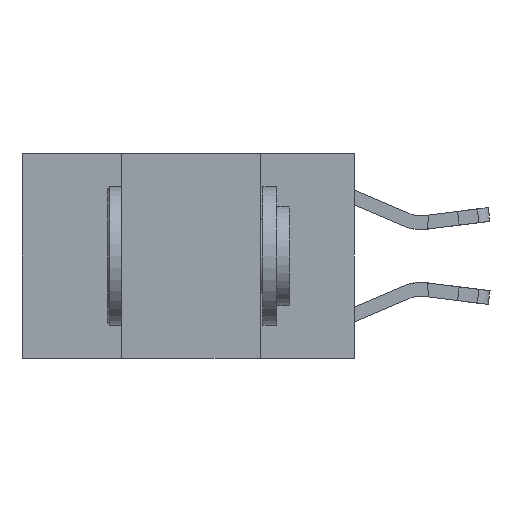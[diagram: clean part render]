
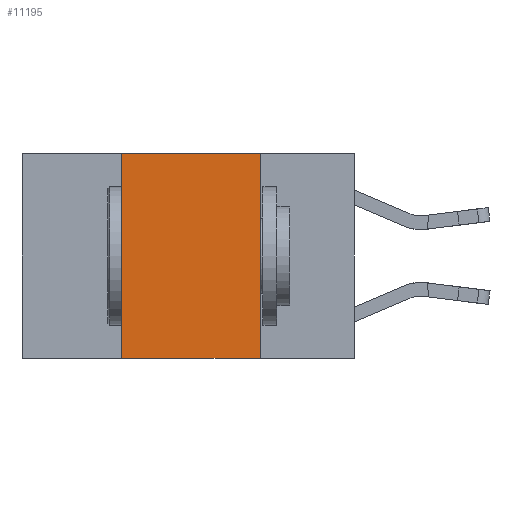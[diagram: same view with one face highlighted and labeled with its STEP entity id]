
A CAD part, left-side view. The second image highlights one B-rep face of the part: STEP entity #11195.
In plain terms, the highlighted planar face has unit normal (-1, 0, 0).
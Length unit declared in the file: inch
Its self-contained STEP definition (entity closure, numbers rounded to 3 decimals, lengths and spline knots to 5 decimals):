
#522 = CARTESIAN_POINT ( 'NONE',  ( 0., 0.42, -0.37 ) ) ;
#808 = VECTOR ( 'NONE', #12189, 39.37008 ) ;
#1566 = EDGE_CURVE ( 'NONE', #13893, #15025, #16848, .T. ) ;
#1718 = DIRECTION ( 'NONE',  ( 0., -1., 0. ) ) ;
#2200 = VECTOR ( 'NONE', #12723, 39.37008 ) ;
#2307 = ORIENTED_EDGE ( 'NONE', *, *, #5535, .F. ) ;
#2450 = EDGE_LOOP ( 'NONE', ( #11611, #2307, #12212, #3860 ) ) ;
#3753 = CARTESIAN_POINT ( 'NONE',  ( 0., 0.42, 0. ) ) ;
#3777 = DIRECTION ( 'NONE',  ( 0., 0., 1. ) ) ;
#3816 = EDGE_CURVE ( 'NONE', #8434, #16528, #4394, .T. ) ;
#3860 = ORIENTED_EDGE ( 'NONE', *, *, #13163, .T. ) ;
#4394 = LINE ( 'NONE', #14783, #808 ) ;
#5535 = EDGE_CURVE ( 'NONE', #15025, #8434, #9265, .T. ) ;
#6789 = PLANE ( 'NONE',  #6820 ) ;
#6820 = AXIS2_PLACEMENT_3D ( 'NONE', #10739, #16024, #8118 ) ;
#7435 = CARTESIAN_POINT ( 'NONE',  ( 0., 0.6, 0. ) ) ;
#8118 = DIRECTION ( 'NONE',  ( 0., 0., -1. ) ) ;
#8310 = CARTESIAN_POINT ( 'NONE',  ( 0., 0.17, 0. ) ) ;
#8342 = CARTESIAN_POINT ( 'NONE',  ( 0., 0.6, -0.37 ) ) ;
#8386 = LINE ( 'NONE', #8342, #11094 ) ;
#8434 = VERTEX_POINT ( 'NONE', #8310 ) ;
#9265 = LINE ( 'NONE', #7435, #2200 ) ;
#9804 = CARTESIAN_POINT ( 'NONE',  ( 0., 0.17, -0.37 ) ) ;
#9836 = VECTOR ( 'NONE', #3777, 39.37008 ) ;
#10739 = CARTESIAN_POINT ( 'NONE',  ( 0., 0.6, 0. ) ) ;
#10906 = CARTESIAN_POINT ( 'NONE',  ( 0., 0.42, 0. ) ) ;
#11094 = VECTOR ( 'NONE', #1718, 39.37008 ) ;
#11195 = ADVANCED_FACE ( 'NONE', ( #16303 ), #6789, .F. ) ;
#11611 = ORIENTED_EDGE ( 'NONE', *, *, #3816, .F. ) ;
#12189 = DIRECTION ( 'NONE',  ( 0., 0., -1. ) ) ;
#12212 = ORIENTED_EDGE ( 'NONE', *, *, #1566, .F. ) ;
#12723 = DIRECTION ( 'NONE',  ( 0., -1., 0. ) ) ;
#13163 = EDGE_CURVE ( 'NONE', #13893, #16528, #8386, .T. ) ;
#13893 = VERTEX_POINT ( 'NONE', #522 ) ;
#14783 = CARTESIAN_POINT ( 'NONE',  ( 0., 0.17, 0. ) ) ;
#15025 = VERTEX_POINT ( 'NONE', #10906 ) ;
#16024 = DIRECTION ( 'NONE',  ( 1., 0., 0. ) ) ;
#16303 = FACE_OUTER_BOUND ( 'NONE', #2450, .T. ) ;
#16528 = VERTEX_POINT ( 'NONE', #9804 ) ;
#16848 = LINE ( 'NONE', #3753, #9836 ) ;
